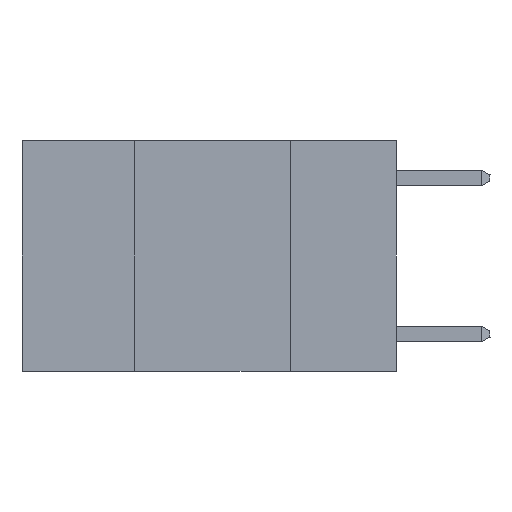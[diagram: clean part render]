
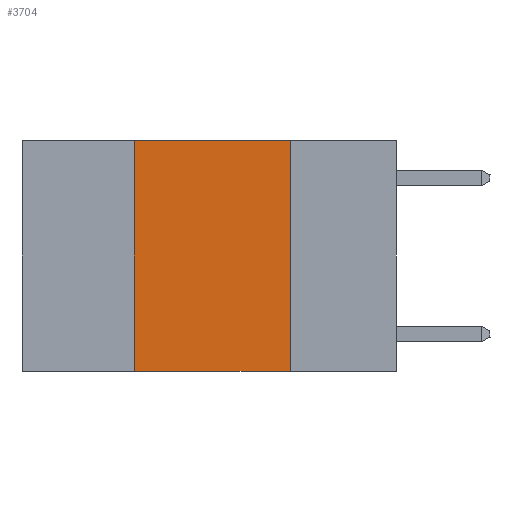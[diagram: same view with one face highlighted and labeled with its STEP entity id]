
A CAD part, left-side view. The second image highlights one B-rep face of the part: STEP entity #3704.
In plain terms, the highlighted planar face has unit normal (-1, 0, 0).
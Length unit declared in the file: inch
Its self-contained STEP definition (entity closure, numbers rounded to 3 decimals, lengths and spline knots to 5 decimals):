
#261 = ORIENTED_EDGE ( 'NONE', *, *, #10317, .F. ) ;
#1519 = CARTESIAN_POINT ( 'NONE',  ( 0., 0.6, 0. ) ) ;
#2834 = DIRECTION ( 'NONE',  ( 0., 0., -1. ) ) ;
#3704 = ADVANCED_FACE ( 'NONE', ( #13949 ), #20163, .F. ) ;
#3866 = ORIENTED_EDGE ( 'NONE', *, *, #17891, .F. ) ;
#4424 = LINE ( 'NONE', #13868, #12060 ) ;
#5402 = LINE ( 'NONE', #11668, #10668 ) ;
#5606 = DIRECTION ( 'NONE',  ( 0., -1., 0. ) ) ;
#6225 = DIRECTION ( 'NONE',  ( 1., 0., 0. ) ) ;
#6890 = CARTESIAN_POINT ( 'NONE',  ( 0., 0.17, 0. ) ) ;
#7135 = AXIS2_PLACEMENT_3D ( 'NONE', #1519, #6225, #2834 ) ;
#7351 = DIRECTION ( 'NONE',  ( 0., 0., -1. ) ) ;
#7430 = ORIENTED_EDGE ( 'NONE', *, *, #15948, .T. ) ;
#7568 = CARTESIAN_POINT ( 'NONE',  ( 0., 0.17, 0. ) ) ;
#8793 = CARTESIAN_POINT ( 'NONE',  ( 0., 0.42, -0.37 ) ) ;
#9019 = LINE ( 'NONE', #7568, #17856 ) ;
#10317 = EDGE_CURVE ( 'NONE', #18050, #10683, #18261, .T. ) ;
#10668 = VECTOR ( 'NONE', #5606, 39.37008 ) ;
#10683 = VERTEX_POINT ( 'NONE', #6890 ) ;
#11076 = CARTESIAN_POINT ( 'NONE',  ( 0., 0.42, 0. ) ) ;
#11668 = CARTESIAN_POINT ( 'NONE',  ( 0., 0.6, -0.37 ) ) ;
#12060 = VECTOR ( 'NONE', #20084, 39.37008 ) ;
#12088 = CARTESIAN_POINT ( 'NONE',  ( 0., 0.17, -0.37 ) ) ;
#13487 = EDGE_LOOP ( 'NONE', ( #3866, #261, #16635, #7430 ) ) ;
#13868 = CARTESIAN_POINT ( 'NONE',  ( 0., 0.42, 0. ) ) ;
#13949 = FACE_OUTER_BOUND ( 'NONE', #13487, .T. ) ;
#14507 = VERTEX_POINT ( 'NONE', #8793 ) ;
#15532 = VERTEX_POINT ( 'NONE', #12088 ) ;
#15948 = EDGE_CURVE ( 'NONE', #14507, #15532, #5402, .T. ) ;
#16635 = ORIENTED_EDGE ( 'NONE', *, *, #18328, .F. ) ;
#17022 = VECTOR ( 'NONE', #19992, 39.37008 ) ;
#17856 = VECTOR ( 'NONE', #7351, 39.37008 ) ;
#17891 = EDGE_CURVE ( 'NONE', #10683, #15532, #9019, .T. ) ;
#18050 = VERTEX_POINT ( 'NONE', #11076 ) ;
#18261 = LINE ( 'NONE', #19887, #17022 ) ;
#18328 = EDGE_CURVE ( 'NONE', #14507, #18050, #4424, .T. ) ;
#19887 = CARTESIAN_POINT ( 'NONE',  ( 0., 0.6, 0. ) ) ;
#19992 = DIRECTION ( 'NONE',  ( 0., -1., 0. ) ) ;
#20084 = DIRECTION ( 'NONE',  ( 0., 0., 1. ) ) ;
#20163 = PLANE ( 'NONE',  #7135 ) ;
